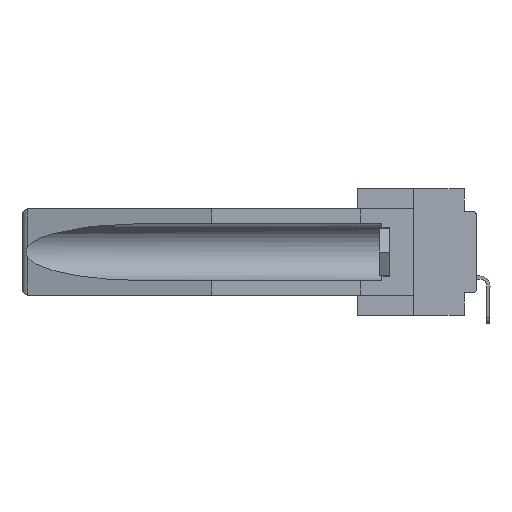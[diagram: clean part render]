
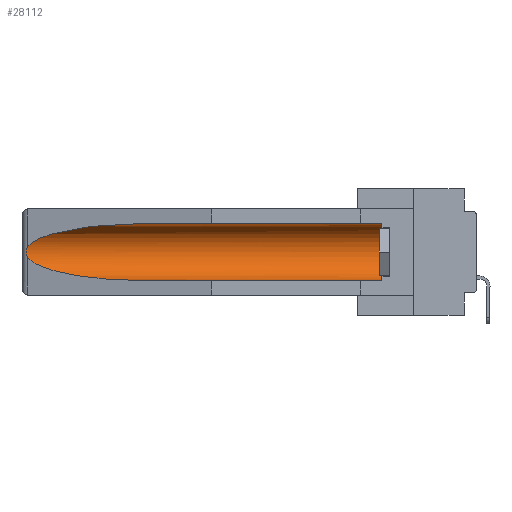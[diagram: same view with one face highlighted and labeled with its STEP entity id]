
A CAD part, left-side view. The second image highlights one B-rep face of the part: STEP entity #28112.
In plain terms, the highlighted cylindrical face has radius 2.857 mm (diameter 5.715 mm), a partial arc.
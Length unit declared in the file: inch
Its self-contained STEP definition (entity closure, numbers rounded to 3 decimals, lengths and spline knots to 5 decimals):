
#221 = VERTEX_POINT ( 'NONE', #26254 ) ;
#411 = EDGE_CURVE ( 'NONE', #27897, #23040, #25437, .T. ) ;
#2186 = AXIS2_PLACEMENT_3D ( 'NONE', #20622, #8863, #25240 ) ;
#2681 = LINE ( 'NONE', #12409, #3802 ) ;
#3298 = CARTESIAN_POINT ( 'NONE',  ( 0.25451, 1.48313, -0.24835 ) ) ;
#3490 = CARTESIAN_POINT ( 'NONE',  ( 0.2673, 1.5327, -0.16383 ) ) ;
#3693 = CARTESIAN_POINT ( 'NONE',  ( 0.26597, 1.52961, -0.15275 ) ) ;
#3802 = VECTOR ( 'NONE', #17041, 39.37008 ) ;
#3944 = CARTESIAN_POINT ( 'NONE',  ( 0.26537, 1.52718, -0.14972 ) ) ;
#5209 = CARTESIAN_POINT ( 'NONE',  ( 0.155, 0.126, -0.1715 ) ) ;
#6385 = EDGE_CURVE ( 'NONE', #221, #23040, #2681, .T. ) ;
#7156 = VERTEX_POINT ( 'NONE', #17634 ) ;
#7216 = EDGE_CURVE ( 'NONE', #7156, #15450, #26969, .T. ) ;
#7674 = VERTEX_POINT ( 'NONE', #29831 ) ;
#8863 = DIRECTION ( 'NONE',  ( 0., 1., 0. ) ) ;
#9557 = DIRECTION ( 'NONE',  ( 0., 0., 1. ) ) ;
#9577 = EDGE_CURVE ( 'NONE', #7674, #27897, #30332, .T. ) ;
#10486 = CARTESIAN_POINT ( 'NONE',  ( 0.155, 1.07973, -0.284 ) ) ;
#10896 = CARTESIAN_POINT ( 'NONE',  ( 0.26597, 1.5296, -0.19026 ) ) ;
#12409 = CARTESIAN_POINT ( 'NONE',  ( 0.155, -0.30754, -0.284 ) ) ;
#12750 = CARTESIAN_POINT ( 'NONE',  ( 0.21114, 1.30732, -0.284 ) ) ;
#12962 = CARTESIAN_POINT ( 'NONE',  ( 0.2675, 1.53308, -0.17534 ) ) ;
#13163 = CARTESIAN_POINT ( 'NONE',  ( 0.2675, 1.53308, -0.16763 ) ) ;
#13405 = ORIENTED_EDGE ( 'NONE', *, *, #14762, .T. ) ;
#14762 = EDGE_CURVE ( 'NONE', #221, #7156, #24056, .T. ) ;
#15446 = CARTESIAN_POINT ( 'NONE',  ( 0.26655, 1.53094, -0.18657 ) ) ;
#15450 = VERTEX_POINT ( 'NONE', #28965 ) ;
#16806 = CARTESIAN_POINT ( 'NONE',  ( 0.155, 1.07973, -0.284 ) ) ;
#17041 = DIRECTION ( 'NONE',  ( 0., 1., 0. ) ) ;
#17577 = FACE_OUTER_BOUND ( 'NONE', #27732, .T. ) ;
#17634 = CARTESIAN_POINT ( 'NONE',  ( 0.155, 0.126, -0.059 ) ) ;
#18001 = CARTESIAN_POINT ( 'NONE',  ( 0.2673, 1.53269, -0.17917 ) ) ;
#18457 = ORIENTED_EDGE ( 'NONE', *, *, #23264, .T. ) ;
#18705 = ORIENTED_EDGE ( 'NONE', *, *, #9577, .T. ) ;
#19809 = CARTESIAN_POINT ( 'NONE',  ( 0.155, 1.07973, -0.059 ) ) ;
#20237 = CARTESIAN_POINT ( 'NONE',  ( 0.25451, 1.48313, -0.09465 ) ) ;
#20622 = CARTESIAN_POINT ( 'NONE',  ( 0.155, -0.30754, -0.1715 ) ) ;
#21067 = VECTOR ( 'NONE', #27719, 39.37008 ) ;
#21769 = ORIENTED_EDGE ( 'NONE', *, *, #6385, .F. ) ;
#22294 = CARTESIAN_POINT ( 'NONE',  ( 0.21114, 1.30732, -0.059 ) ) ;
#22497 = CARTESIAN_POINT ( 'NONE',  ( 0.155, -0.30754, -0.059 ) ) ;
#23040 = VERTEX_POINT ( 'NONE', #16806 ) ;
#23264 = EDGE_CURVE ( 'NONE', #15450, #7674, #29949, .T. ) ;
#24056 = CIRCLE ( 'NONE', #30297, 0.1125 ) ;
#24587 = CARTESIAN_POINT ( 'NONE',  ( 0.26537, 1.52718, -0.19328 ) ) ;
#24593 = CARTESIAN_POINT ( 'NONE',  ( 0.26537, 1.52718, -0.19328 ) ) ;
#24931 = CARTESIAN_POINT ( 'NONE',  ( 0.26537, 1.52718, -0.19328 ) ) ;
#24993 = CARTESIAN_POINT ( 'NONE',  ( 0.26654, 1.53092, -0.15636 ) ) ;
#25240 = DIRECTION ( 'NONE',  ( 0., 0., 1. ) ) ;
#25332 = CYLINDRICAL_SURFACE ( 'NONE', #2186, 0.1125 ) ;
#25437 =( BOUNDED_CURVE ( )  B_SPLINE_CURVE ( 3, ( #24593, #3298, #12750, #10486 ),
 .UNSPECIFIED., .F., .F. ) 
 B_SPLINE_CURVE_WITH_KNOTS ( ( 4, 4 ),
 ( 0.1948, 1.5708 ),
 .UNSPECIFIED. ) 
 CURVE ( )  GEOMETRIC_REPRESENTATION_ITEM ( )  RATIONAL_B_SPLINE_CURVE ( ( 1., 0.848, 0.848, 1. ) ) 
 REPRESENTATION_ITEM ( '' )  );
#26254 = CARTESIAN_POINT ( 'NONE',  ( 0.155, 0.126, -0.284 ) ) ;
#26969 = LINE ( 'NONE', #22497, #21067 ) ;
#27719 = DIRECTION ( 'NONE',  ( 0., 1., 0. ) ) ;
#27732 = EDGE_LOOP ( 'NONE', ( #18457, #18705, #28287, #21769, #13405, #27782 ) ) ;
#27782 = ORIENTED_EDGE ( 'NONE', *, *, #7216, .T. ) ;
#27897 = VERTEX_POINT ( 'NONE', #24931 ) ;
#28112 = ADVANCED_FACE ( 'NONE', ( #17577 ), #25332, .F. ) ;
#28287 = ORIENTED_EDGE ( 'NONE', *, *, #411, .T. ) ;
#28691 = DIRECTION ( 'NONE',  ( 0., -1., 0. ) ) ;
#28965 = CARTESIAN_POINT ( 'NONE',  ( 0.155, 1.07973, -0.059 ) ) ;
#29526 = CARTESIAN_POINT ( 'NONE',  ( 0.26537, 1.52718, -0.14972 ) ) ;
#29831 = CARTESIAN_POINT ( 'NONE',  ( 0.26537, 1.52718, -0.14972 ) ) ;
#29949 =( BOUNDED_CURVE ( )  B_SPLINE_CURVE ( 3, ( #19809, #22294, #20237, #3944 ),
 .UNSPECIFIED., .F., .F. ) 
 B_SPLINE_CURVE_WITH_KNOTS ( ( 4, 4 ),
 ( 4.71239, 6.08839 ),
 .UNSPECIFIED. ) 
 CURVE ( )  GEOMETRIC_REPRESENTATION_ITEM ( )  RATIONAL_B_SPLINE_CURVE ( ( 1., 0.848, 0.848, 1. ) ) 
 REPRESENTATION_ITEM ( '' )  );
#30297 = AXIS2_PLACEMENT_3D ( 'NONE', #5209, #28691, #9557 ) ;
#30332 = B_SPLINE_CURVE_WITH_KNOTS ( 'NONE', 3,
 ( #29526, #3693, #24993, #3490, #13163, #12962, #18001, #15446, #10896, #24587 ),
 .UNSPECIFIED., .F., .F.,
 ( 4, 2, 2, 2, 4 ),
 ( 0., 0.00029, 0.00058, 0.00087, 0.00117 ),
 .UNSPECIFIED. ) ;
